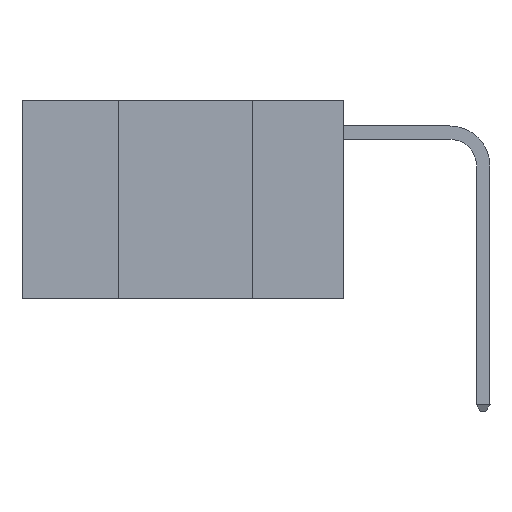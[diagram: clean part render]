
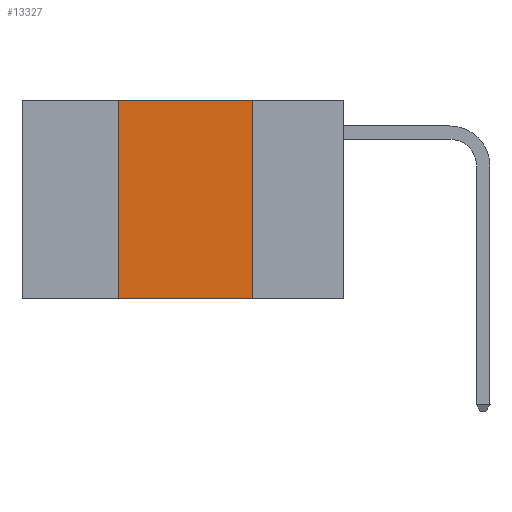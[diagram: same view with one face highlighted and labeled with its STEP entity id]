
A CAD part, left-side view. The second image highlights one B-rep face of the part: STEP entity #13327.
In plain terms, the highlighted planar face has unit normal (-1, 0, 0).
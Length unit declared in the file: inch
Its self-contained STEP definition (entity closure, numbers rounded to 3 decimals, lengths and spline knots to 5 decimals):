
#1629 = VERTEX_POINT ( 'NONE', #5892 ) ;
#1676 = DIRECTION ( 'NONE',  ( 0., 0., -1. ) ) ;
#1827 = VERTEX_POINT ( 'NONE', #28587 ) ;
#1954 = VECTOR ( 'NONE', #17894, 39.37008 ) ;
#3162 = DIRECTION ( 'NONE',  ( 1., 0., 0. ) ) ;
#4231 = VECTOR ( 'NONE', #22319, 39.37008 ) ;
#4351 = CARTESIAN_POINT ( 'NONE',  ( 0., 0.6, -0.37 ) ) ;
#4971 = EDGE_CURVE ( 'NONE', #25030, #1629, #25630, .T. ) ;
#5892 = CARTESIAN_POINT ( 'NONE',  ( 0., 0.42, 0. ) ) ;
#8416 = CARTESIAN_POINT ( 'NONE',  ( 0., 0.17, 0. ) ) ;
#9392 = EDGE_CURVE ( 'NONE', #1629, #22074, #16250, .T. ) ;
#11089 = ORIENTED_EDGE ( 'NONE', *, *, #27447, .T. ) ;
#12003 = EDGE_LOOP ( 'NONE', ( #21700, #16401, #28330, #11089 ) ) ;
#13327 = ADVANCED_FACE ( 'NONE', ( #15633 ), #16720, .F. ) ;
#14580 = CARTESIAN_POINT ( 'NONE',  ( 0., 0.42, -0.37 ) ) ;
#15393 = LINE ( 'NONE', #4351, #1954 ) ;
#15633 = FACE_OUTER_BOUND ( 'NONE', #12003, .T. ) ;
#16250 = LINE ( 'NONE', #17783, #4231 ) ;
#16370 = AXIS2_PLACEMENT_3D ( 'NONE', #21146, #3162, #18971 ) ;
#16401 = ORIENTED_EDGE ( 'NONE', *, *, #9392, .F. ) ;
#16720 = PLANE ( 'NONE',  #16370 ) ;
#17739 = EDGE_CURVE ( 'NONE', #22074, #1827, #28787, .T. ) ;
#17783 = CARTESIAN_POINT ( 'NONE',  ( 0., 0.6, 0. ) ) ;
#17894 = DIRECTION ( 'NONE',  ( 0., -1., 0. ) ) ;
#18579 = DIRECTION ( 'NONE',  ( 0., 0., 1. ) ) ;
#18971 = DIRECTION ( 'NONE',  ( 0., 0., -1. ) ) ;
#21146 = CARTESIAN_POINT ( 'NONE',  ( 0., 0.6, 0. ) ) ;
#21700 = ORIENTED_EDGE ( 'NONE', *, *, #17739, .F. ) ;
#22074 = VERTEX_POINT ( 'NONE', #23794 ) ;
#22319 = DIRECTION ( 'NONE',  ( 0., -1., 0. ) ) ;
#22864 = VECTOR ( 'NONE', #1676, 39.37008 ) ;
#23794 = CARTESIAN_POINT ( 'NONE',  ( 0., 0.17, 0. ) ) ;
#24232 = VECTOR ( 'NONE', #18579, 39.37008 ) ;
#25030 = VERTEX_POINT ( 'NONE', #14580 ) ;
#25630 = LINE ( 'NONE', #27478, #24232 ) ;
#27447 = EDGE_CURVE ( 'NONE', #25030, #1827, #15393, .T. ) ;
#27478 = CARTESIAN_POINT ( 'NONE',  ( 0., 0.42, 0. ) ) ;
#28330 = ORIENTED_EDGE ( 'NONE', *, *, #4971, .F. ) ;
#28587 = CARTESIAN_POINT ( 'NONE',  ( 0., 0.17, -0.37 ) ) ;
#28787 = LINE ( 'NONE', #8416, #22864 ) ;
